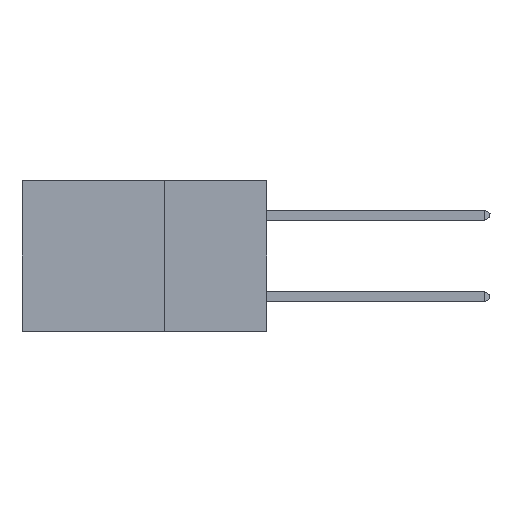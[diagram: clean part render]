
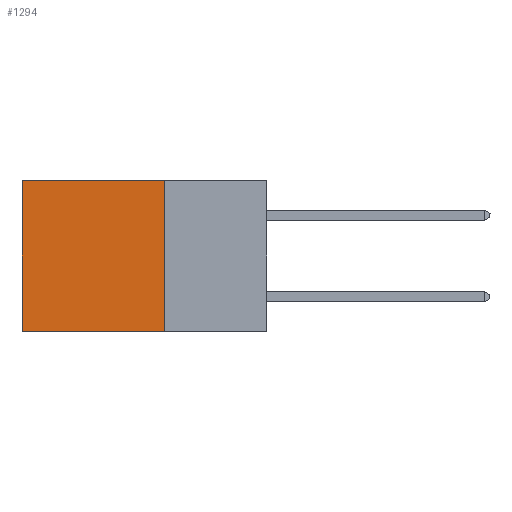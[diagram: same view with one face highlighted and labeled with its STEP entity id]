
A CAD part, left-side view. The second image highlights one B-rep face of the part: STEP entity #1294.
In plain terms, the highlighted planar face has unit normal (-1, 0, 0).
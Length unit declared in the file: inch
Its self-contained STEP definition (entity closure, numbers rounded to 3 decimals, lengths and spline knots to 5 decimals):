
#504 = LINE ( 'NONE', #5359, #10902 ) ;
#583 = VERTEX_POINT ( 'NONE', #3758 ) ;
#900 = VERTEX_POINT ( 'NONE', #11589 ) ;
#941 = LINE ( 'NONE', #8688, #6187 ) ;
#1231 = CARTESIAN_POINT ( 'NONE',  ( 0.2875, 0.25, 0. ) ) ;
#1294 = ADVANCED_FACE ( 'NONE', ( #11943 ), #8297, .F. ) ;
#1493 = VECTOR ( 'NONE', #4184, 39.37008 ) ;
#1803 = EDGE_CURVE ( 'NONE', #583, #8742, #12063, .T. ) ;
#3758 = CARTESIAN_POINT ( 'NONE',  ( 0.2875, 0.25, 0. ) ) ;
#3959 = AXIS2_PLACEMENT_3D ( 'NONE', #8335, #8630, #9528 ) ;
#4184 = DIRECTION ( 'NONE',  ( 0., 1., 0. ) ) ;
#5302 = ORIENTED_EDGE ( 'NONE', *, *, #8367, .T. ) ;
#5359 = CARTESIAN_POINT ( 'NONE',  ( 0.2875, 0.6, 0. ) ) ;
#5531 = ORIENTED_EDGE ( 'NONE', *, *, #6504, .F. ) ;
#5763 = ORIENTED_EDGE ( 'NONE', *, *, #11371, .F. ) ;
#6187 = VECTOR ( 'NONE', #7755, 39.37008 ) ;
#6504 = EDGE_CURVE ( 'NONE', #900, #7135, #10631, .T. ) ;
#7135 = VERTEX_POINT ( 'NONE', #10461 ) ;
#7153 = ORIENTED_EDGE ( 'NONE', *, *, #1803, .T. ) ;
#7356 = DIRECTION ( 'NONE',  ( 0., 0., -1. ) ) ;
#7733 = DIRECTION ( 'NONE',  ( 0., 1., 0. ) ) ;
#7755 = DIRECTION ( 'NONE',  ( 0., 0., -1. ) ) ;
#8106 = VECTOR ( 'NONE', #7733, 39.37008 ) ;
#8297 = PLANE ( 'NONE',  #3959 ) ;
#8335 = CARTESIAN_POINT ( 'NONE',  ( 0.2875, 0.25, 0. ) ) ;
#8367 = EDGE_CURVE ( 'NONE', #8742, #7135, #504, .T. ) ;
#8630 = DIRECTION ( 'NONE',  ( 1., 0., 0. ) ) ;
#8688 = CARTESIAN_POINT ( 'NONE',  ( 0.2875, 0.25, 0. ) ) ;
#8742 = VERTEX_POINT ( 'NONE', #12477 ) ;
#9528 = DIRECTION ( 'NONE',  ( 0., 0., -1. ) ) ;
#10461 = CARTESIAN_POINT ( 'NONE',  ( 0.2875, 0.6, -0.37 ) ) ;
#10605 = EDGE_LOOP ( 'NONE', ( #5302, #5531, #5763, #7153 ) ) ;
#10631 = LINE ( 'NONE', #11533, #8106 ) ;
#10902 = VECTOR ( 'NONE', #7356, 39.37008 ) ;
#11371 = EDGE_CURVE ( 'NONE', #583, #900, #941, .T. ) ;
#11533 = CARTESIAN_POINT ( 'NONE',  ( 0.2875, 0.25, -0.37 ) ) ;
#11589 = CARTESIAN_POINT ( 'NONE',  ( 0.2875, 0.25, -0.37 ) ) ;
#11943 = FACE_OUTER_BOUND ( 'NONE', #10605, .T. ) ;
#12063 = LINE ( 'NONE', #1231, #1493 ) ;
#12477 = CARTESIAN_POINT ( 'NONE',  ( 0.2875, 0.6, 0. ) ) ;
